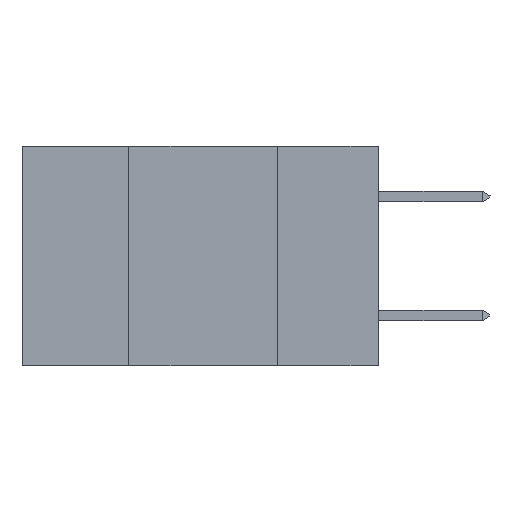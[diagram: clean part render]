
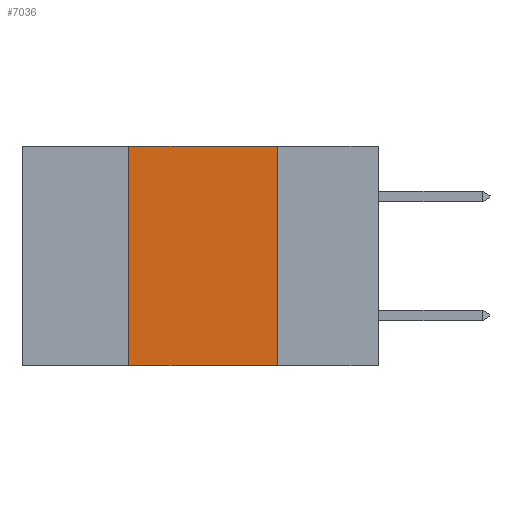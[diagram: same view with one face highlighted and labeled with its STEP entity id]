
A CAD part, left-side view. The second image highlights one B-rep face of the part: STEP entity #7036.
In plain terms, the highlighted planar face has unit normal (-1, 0, 0).
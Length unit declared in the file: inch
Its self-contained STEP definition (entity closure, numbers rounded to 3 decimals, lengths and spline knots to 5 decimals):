
#220 = PLANE ( 'NONE',  #11658 ) ;
#547 = CARTESIAN_POINT ( 'NONE',  ( 0., 0.6, 0. ) ) ;
#591 = EDGE_LOOP ( 'NONE', ( #953, #7964, #14754, #18198 ) ) ;
#953 = ORIENTED_EDGE ( 'NONE', *, *, #20535, .F. ) ;
#2264 = VECTOR ( 'NONE', #2475, 39.37008 ) ;
#2475 = DIRECTION ( 'NONE',  ( 0., 0., -1. ) ) ;
#3068 = VECTOR ( 'NONE', #18145, 39.37008 ) ;
#3685 = DIRECTION ( 'NONE',  ( 0., 0., 1. ) ) ;
#6527 = VECTOR ( 'NONE', #18186, 39.37008 ) ;
#6621 = LINE ( 'NONE', #19976, #6527 ) ;
#7036 = ADVANCED_FACE ( 'NONE', ( #17694 ), #220, .F. ) ;
#7052 = VERTEX_POINT ( 'NONE', #7390 ) ;
#7128 = EDGE_CURVE ( 'NONE', #8857, #7052, #21418, .T. ) ;
#7390 = CARTESIAN_POINT ( 'NONE',  ( 0., 0.17, -0.37 ) ) ;
#7964 = ORIENTED_EDGE ( 'NONE', *, *, #21428, .F. ) ;
#8452 = CARTESIAN_POINT ( 'NONE',  ( 0., 0.42, 0. ) ) ;
#8618 = EDGE_CURVE ( 'NONE', #8857, #8871, #12194, .T. ) ;
#8857 = VERTEX_POINT ( 'NONE', #15158 ) ;
#8871 = VERTEX_POINT ( 'NONE', #8452 ) ;
#11403 = CARTESIAN_POINT ( 'NONE',  ( 0., 0.6, -0.37 ) ) ;
#11658 = AXIS2_PLACEMENT_3D ( 'NONE', #547, #16016, #18941 ) ;
#12194 = LINE ( 'NONE', #13761, #17042 ) ;
#12651 = CARTESIAN_POINT ( 'NONE',  ( 0., 0.17, -0.37 ) ) ;
#13761 = CARTESIAN_POINT ( 'NONE',  ( 0., 0.42, -0.37 ) ) ;
#14754 = ORIENTED_EDGE ( 'NONE', *, *, #8618, .F. ) ;
#15158 = CARTESIAN_POINT ( 'NONE',  ( 0., 0.42, -0.37 ) ) ;
#15815 = VERTEX_POINT ( 'NONE', #19619 ) ;
#16016 = DIRECTION ( 'NONE',  ( 1., 0., 0. ) ) ;
#16125 = LINE ( 'NONE', #12651, #2264 ) ;
#17042 = VECTOR ( 'NONE', #3685, 39.37008 ) ;
#17694 = FACE_OUTER_BOUND ( 'NONE', #591, .T. ) ;
#18145 = DIRECTION ( 'NONE',  ( 0., -1., 0. ) ) ;
#18186 = DIRECTION ( 'NONE',  ( 0., -1., 0. ) ) ;
#18198 = ORIENTED_EDGE ( 'NONE', *, *, #7128, .T. ) ;
#18941 = DIRECTION ( 'NONE',  ( 0., 0., -1. ) ) ;
#19619 = CARTESIAN_POINT ( 'NONE',  ( 0., 0.17, 0. ) ) ;
#19976 = CARTESIAN_POINT ( 'NONE',  ( 0., 0.6, 0. ) ) ;
#20535 = EDGE_CURVE ( 'NONE', #15815, #7052, #16125, .T. ) ;
#21418 = LINE ( 'NONE', #11403, #3068 ) ;
#21428 = EDGE_CURVE ( 'NONE', #8871, #15815, #6621, .T. ) ;
